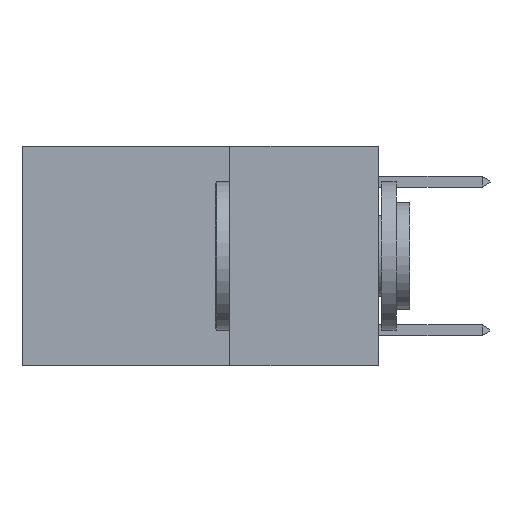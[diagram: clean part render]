
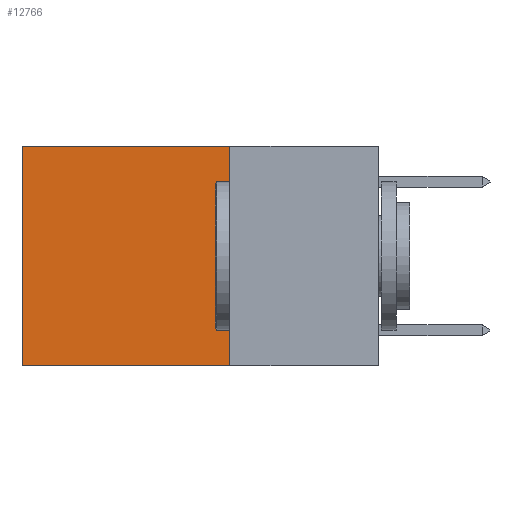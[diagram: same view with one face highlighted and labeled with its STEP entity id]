
A CAD part, left-side view. The second image highlights one B-rep face of the part: STEP entity #12766.
In plain terms, the highlighted planar face has unit normal (-1, 0, 0).
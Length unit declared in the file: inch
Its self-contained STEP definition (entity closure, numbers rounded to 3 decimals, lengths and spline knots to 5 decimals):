
#818 = ORIENTED_EDGE ( 'NONE', *, *, #1038, .T. ) ;
#1038 = EDGE_CURVE ( 'NONE', #13107, #5813, #10504, .T. ) ;
#1991 = CARTESIAN_POINT ( 'NONE',  ( 0.2625, 0.25, 0. ) ) ;
#3204 = LINE ( 'NONE', #10360, #14022 ) ;
#3619 = CARTESIAN_POINT ( 'NONE',  ( 0.2625, 0.6, -0.37 ) ) ;
#3915 = EDGE_CURVE ( 'NONE', #5813, #14552, #3204, .T. ) ;
#4261 = ORIENTED_EDGE ( 'NONE', *, *, #6503, .F. ) ;
#5021 = DIRECTION ( 'NONE',  ( 1., 0., 0. ) ) ;
#5240 = EDGE_LOOP ( 'NONE', ( #15175, #4261, #8830, #818 ) ) ;
#5670 = EDGE_CURVE ( 'NONE', #13107, #12030, #9600, .T. ) ;
#5813 = VERTEX_POINT ( 'NONE', #15437 ) ;
#6503 = EDGE_CURVE ( 'NONE', #12030, #14552, #13906, .T. ) ;
#6929 = CARTESIAN_POINT ( 'NONE',  ( 0.2625, 0.25, -0.37 ) ) ;
#7612 = CARTESIAN_POINT ( 'NONE',  ( 0.2625, 0.25, 0. ) ) ;
#7626 = DIRECTION ( 'NONE',  ( 0., 1., 0. ) ) ;
#8102 = DIRECTION ( 'NONE',  ( 0., 0., -1. ) ) ;
#8312 = FACE_OUTER_BOUND ( 'NONE', #5240, .T. ) ;
#8756 = DIRECTION ( 'NONE',  ( 0., 0., -1. ) ) ;
#8830 = ORIENTED_EDGE ( 'NONE', *, *, #5670, .F. ) ;
#9600 = LINE ( 'NONE', #7612, #12812 ) ;
#9864 = PLANE ( 'NONE',  #13127 ) ;
#10021 = DIRECTION ( 'NONE',  ( 0., 0., -1. ) ) ;
#10360 = CARTESIAN_POINT ( 'NONE',  ( 0.2625, 0.6, 0. ) ) ;
#10504 = LINE ( 'NONE', #12288, #13919 ) ;
#11064 = CARTESIAN_POINT ( 'NONE',  ( 0.2625, 0.25, 0. ) ) ;
#12030 = VERTEX_POINT ( 'NONE', #6929 ) ;
#12288 = CARTESIAN_POINT ( 'NONE',  ( 0.2625, 0.25, 0. ) ) ;
#12766 = ADVANCED_FACE ( 'NONE', ( #8312 ), #9864, .F. ) ;
#12812 = VECTOR ( 'NONE', #10021, 39.37008 ) ;
#13107 = VERTEX_POINT ( 'NONE', #1991 ) ;
#13127 = AXIS2_PLACEMENT_3D ( 'NONE', #11064, #5021, #8756 ) ;
#13343 = CARTESIAN_POINT ( 'NONE',  ( 0.2625, 0.25, -0.37 ) ) ;
#13874 = VECTOR ( 'NONE', #15730, 39.37008 ) ;
#13906 = LINE ( 'NONE', #13343, #13874 ) ;
#13919 = VECTOR ( 'NONE', #7626, 39.37008 ) ;
#14022 = VECTOR ( 'NONE', #8102, 39.37008 ) ;
#14552 = VERTEX_POINT ( 'NONE', #3619 ) ;
#15175 = ORIENTED_EDGE ( 'NONE', *, *, #3915, .T. ) ;
#15437 = CARTESIAN_POINT ( 'NONE',  ( 0.2625, 0.6, 0. ) ) ;
#15730 = DIRECTION ( 'NONE',  ( 0., 1., 0. ) ) ;
